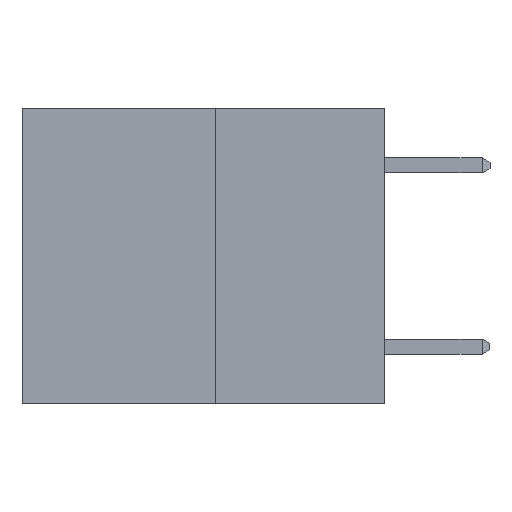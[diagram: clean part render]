
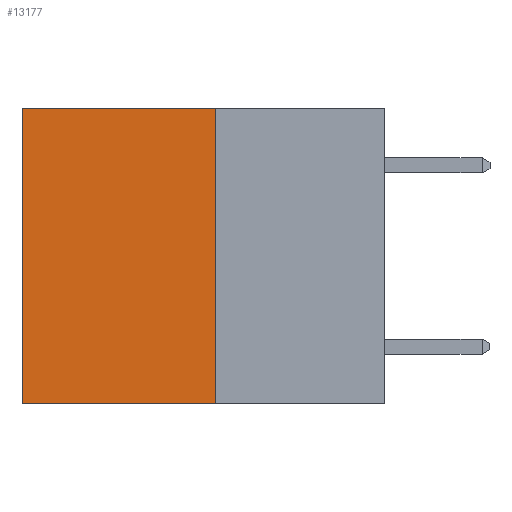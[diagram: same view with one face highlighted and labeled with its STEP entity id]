
A CAD part, left-side view. The second image highlights one B-rep face of the part: STEP entity #13177.
In plain terms, the highlighted planar face has unit normal (-1, 0, 0).
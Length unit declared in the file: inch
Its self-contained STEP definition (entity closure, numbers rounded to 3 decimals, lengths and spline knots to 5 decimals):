
#92 = PLANE ( 'NONE',  #9886 ) ;
#100 = LINE ( 'NONE', #1517, #16419 ) ;
#207 = VECTOR ( 'NONE', #16982, 39.37008 ) ;
#531 = CARTESIAN_POINT ( 'NONE',  ( 0.3165, 0.28, 0. ) ) ;
#561 = EDGE_CURVE ( 'NONE', #14500, #4115, #9837, .T. ) ;
#1517 = CARTESIAN_POINT ( 'NONE',  ( 0.3165, 0.6, -0.49 ) ) ;
#2490 = CARTESIAN_POINT ( 'NONE',  ( 0.3165, 0.28, -0.49 ) ) ;
#2741 = VERTEX_POINT ( 'NONE', #9564 ) ;
#3802 = FACE_OUTER_BOUND ( 'NONE', #3850, .T. ) ;
#3850 = EDGE_LOOP ( 'NONE', ( #6871, #6465, #8243, #9633 ) ) ;
#4115 = VERTEX_POINT ( 'NONE', #6840 ) ;
#4194 = EDGE_CURVE ( 'NONE', #7756, #4115, #100, .T. ) ;
#5351 = CARTESIAN_POINT ( 'NONE',  ( 0.3165, 0.6, 0. ) ) ;
#5570 = DIRECTION ( 'NONE',  ( 0., 0., -1. ) ) ;
#6465 = ORIENTED_EDGE ( 'NONE', *, *, #561, .F. ) ;
#6840 = CARTESIAN_POINT ( 'NONE',  ( 0.3165, 0.6, -0.49 ) ) ;
#6871 = ORIENTED_EDGE ( 'NONE', *, *, #4194, .T. ) ;
#7026 = CARTESIAN_POINT ( 'NONE',  ( 0.3165, 0.28, -0.49 ) ) ;
#7036 = VECTOR ( 'NONE', #12518, 39.37008 ) ;
#7756 = VERTEX_POINT ( 'NONE', #5351 ) ;
#8243 = ORIENTED_EDGE ( 'NONE', *, *, #8723, .F. ) ;
#8671 = DIRECTION ( 'NONE',  ( 0., 1., 0. ) ) ;
#8723 = EDGE_CURVE ( 'NONE', #2741, #14500, #10345, .T. ) ;
#9564 = CARTESIAN_POINT ( 'NONE',  ( 0.3165, 0.28, 0. ) ) ;
#9633 = ORIENTED_EDGE ( 'NONE', *, *, #10505, .T. ) ;
#9837 = LINE ( 'NONE', #14392, #207 ) ;
#9886 = AXIS2_PLACEMENT_3D ( 'NONE', #2490, #11829, #17213 ) ;
#10345 = LINE ( 'NONE', #7026, #7036 ) ;
#10505 = EDGE_CURVE ( 'NONE', #2741, #7756, #13605, .T. ) ;
#10915 = VECTOR ( 'NONE', #8671, 39.37008 ) ;
#11829 = DIRECTION ( 'NONE',  ( 1., 0., 0. ) ) ;
#12518 = DIRECTION ( 'NONE',  ( 0., 0., -1. ) ) ;
#13177 = ADVANCED_FACE ( 'NONE', ( #3802 ), #92, .F. ) ;
#13605 = LINE ( 'NONE', #531, #10915 ) ;
#14392 = CARTESIAN_POINT ( 'NONE',  ( 0.3165, 0.28, -0.49 ) ) ;
#14500 = VERTEX_POINT ( 'NONE', #15598 ) ;
#15598 = CARTESIAN_POINT ( 'NONE',  ( 0.3165, 0.28, -0.49 ) ) ;
#16419 = VECTOR ( 'NONE', #5570, 39.37008 ) ;
#16982 = DIRECTION ( 'NONE',  ( 0., 1., 0. ) ) ;
#17213 = DIRECTION ( 'NONE',  ( 0., 0., -1. ) ) ;
